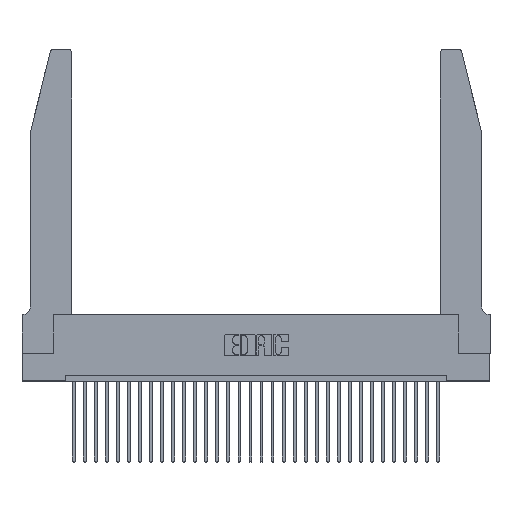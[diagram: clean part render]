
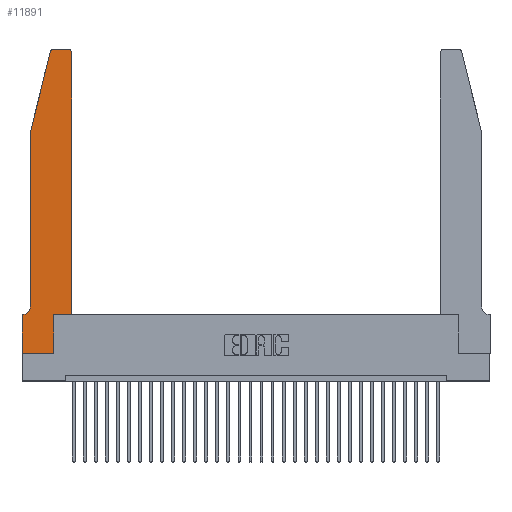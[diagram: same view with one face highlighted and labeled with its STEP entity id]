
A CAD part, top view. The second image highlights one B-rep face of the part: STEP entity #11891.
In plain terms, the highlighted planar face has unit normal (0, 0, 1).
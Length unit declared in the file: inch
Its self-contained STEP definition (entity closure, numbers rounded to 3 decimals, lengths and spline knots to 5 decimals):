
#624 = DIRECTION ( 'NONE',  ( 0., -1., 0. ) ) ;
#939 = EDGE_CURVE ( 'NONE', #3533, #28331, #27100, .T. ) ;
#1488 = EDGE_CURVE ( 'NONE', #28331, #21614, #12310, .T. ) ;
#1603 = VERTEX_POINT ( 'NONE', #28824 ) ;
#1718 = AXIS2_PLACEMENT_3D ( 'NONE', #11492, #25703, #21127 ) ;
#2092 = CARTESIAN_POINT ( 'NONE',  ( 0.0055, 0.35, 0.37 ) ) ;
#2944 = CARTESIAN_POINT ( 'NONE',  ( 0.4505, 0.35, 0.37 ) ) ;
#3262 = VECTOR ( 'NONE', #7074, 39.37008 ) ;
#3434 = AXIS2_PLACEMENT_3D ( 'NONE', #5565, #19455, #17740 ) ;
#3473 = CARTESIAN_POINT ( 'NONE',  ( 0.4505, 2.72, 0.37 ) ) ;
#3480 = ORIENTED_EDGE ( 'NONE', *, *, #20448, .T. ) ;
#3533 = VERTEX_POINT ( 'NONE', #3473 ) ;
#3697 = CARTESIAN_POINT ( 'NONE',  ( 0., 0.35, 0.37 ) ) ;
#4488 = VECTOR ( 'NONE', #15259, 39.37008 ) ;
#5148 = EDGE_CURVE ( 'NONE', #29528, #20978, #16228, .T. ) ;
#5565 = CARTESIAN_POINT ( 'NONE',  ( 0.0055, 0.42, 0.37 ) ) ;
#5737 = CARTESIAN_POINT ( 'NONE',  ( 0., 0., 0.37 ) ) ;
#6694 = ORIENTED_EDGE ( 'NONE', *, *, #939, .T. ) ;
#6777 = CIRCLE ( 'NONE', #3434, 0.07 ) ;
#6950 = EDGE_CURVE ( 'NONE', #27417, #1603, #30986, .T. ) ;
#7074 = DIRECTION ( 'NONE',  ( 0., 1., 0. ) ) ;
#7386 = CARTESIAN_POINT ( 'NONE',  ( 0.4505, 0.35, 0.37 ) ) ;
#7404 = ORIENTED_EDGE ( 'NONE', *, *, #1488, .T. ) ;
#7654 = CIRCLE ( 'NONE', #24157, 0.03 ) ;
#7812 = LINE ( 'NONE', #21998, #14275 ) ;
#8032 = ORIENTED_EDGE ( 'NONE', *, *, #24967, .T. ) ;
#8493 = ORIENTED_EDGE ( 'NONE', *, *, #16739, .T. ) ;
#8572 = CARTESIAN_POINT ( 'NONE',  ( 0.4205, 2.75, 0.37 ) ) ;
#8631 = LINE ( 'NONE', #7386, #3262 ) ;
#8802 = CARTESIAN_POINT ( 'NONE',  ( 0.284, 2.75, 0.37 ) ) ;
#8907 = VECTOR ( 'NONE', #25138, 39.37008 ) ;
#9282 = VERTEX_POINT ( 'NONE', #10250 ) ;
#9800 = EDGE_LOOP ( 'NONE', ( #7404, #21762, #13279, #27563, #30199, #23719, #8493, #3480, #22767, #8032, #12245, #6694 ) ) ;
#9854 = VECTOR ( 'NONE', #624, 39.37008 ) ;
#9991 = CARTESIAN_POINT ( 'NONE',  ( 0.0755, 2., 0.37 ) ) ;
#10250 = CARTESIAN_POINT ( 'NONE',  ( 0.25487, 2.72718, 0.37 ) ) ;
#11074 = CARTESIAN_POINT ( 'NONE',  ( 0.0755, 0.35, 0.37 ) ) ;
#11308 = CARTESIAN_POINT ( 'NONE',  ( 0., 0., 0.37 ) ) ;
#11477 = AXIS2_PLACEMENT_3D ( 'NONE', #28667, #11798, #26436 ) ;
#11492 = CARTESIAN_POINT ( 'NONE',  ( 0.4205, 2.72, 0.37 ) ) ;
#11588 = CARTESIAN_POINT ( 'NONE',  ( 0.284, 2.72, 0.37 ) ) ;
#11798 = DIRECTION ( 'NONE',  ( 0., 0., 1. ) ) ;
#11891 = ADVANCED_FACE ( 'NONE', ( #31187 ), #31394, .T. ) ;
#12128 = VECTOR ( 'NONE', #30871, 39.37008 ) ;
#12245 = ORIENTED_EDGE ( 'NONE', *, *, #24285, .T. ) ;
#12310 = LINE ( 'NONE', #27388, #8907 ) ;
#12819 = VECTOR ( 'NONE', #28152, 39.37008 ) ;
#13279 = ORIENTED_EDGE ( 'NONE', *, *, #23619, .T. ) ;
#13981 = LINE ( 'NONE', #11074, #12819 ) ;
#14224 = CARTESIAN_POINT ( 'NONE',  ( 0.0755, 2., 0.37 ) ) ;
#14275 = VECTOR ( 'NONE', #14578, 39.37008 ) ;
#14578 = DIRECTION ( 'NONE',  ( 1., 0., 0. ) ) ;
#14984 = VERTEX_POINT ( 'NONE', #2092 ) ;
#15259 = DIRECTION ( 'NONE',  ( -0.239, -0.971, 0. ) ) ;
#15843 = LINE ( 'NONE', #9991, #4488 ) ;
#16228 = LINE ( 'NONE', #14224, #12128 ) ;
#16281 = LINE ( 'NONE', #5737, #9854 ) ;
#16739 = EDGE_CURVE ( 'NONE', #27795, #19474, #16281, .T. ) ;
#17278 = EDGE_CURVE ( 'NONE', #21614, #9282, #7654, .T. ) ;
#17740 = DIRECTION ( 'NONE',  ( -1., 0., 0. ) ) ;
#18442 = DIRECTION ( 'NONE',  ( 0., 1., 0. ) ) ;
#19332 = VECTOR ( 'NONE', #19713, 39.37008 ) ;
#19455 = DIRECTION ( 'NONE',  ( 0., 0., -1. ) ) ;
#19474 = VERTEX_POINT ( 'NONE', #11308 ) ;
#19713 = DIRECTION ( 'NONE',  ( 1., 0., 0. ) ) ;
#19762 = EDGE_CURVE ( 'NONE', #20978, #14984, #6777, .T. ) ;
#20448 = EDGE_CURVE ( 'NONE', #19474, #27417, #30721, .T. ) ;
#20576 = CARTESIAN_POINT ( 'NONE',  ( 0.0755, 2., 0.37 ) ) ;
#20978 = VERTEX_POINT ( 'NONE', #25087 ) ;
#21127 = DIRECTION ( 'NONE',  ( 1., 0., 0. ) ) ;
#21462 = CARTESIAN_POINT ( 'NONE',  ( 0.2865, 0., 0.37 ) ) ;
#21614 = VERTEX_POINT ( 'NONE', #8802 ) ;
#21762 = ORIENTED_EDGE ( 'NONE', *, *, #17278, .T. ) ;
#21998 = CARTESIAN_POINT ( 'NONE',  ( 0.4505, 0.35, 0.37 ) ) ;
#22229 = VECTOR ( 'NONE', #18442, 39.37008 ) ;
#22767 = ORIENTED_EDGE ( 'NONE', *, *, #6950, .T. ) ;
#23619 = EDGE_CURVE ( 'NONE', #9282, #29528, #15843, .T. ) ;
#23719 = ORIENTED_EDGE ( 'NONE', *, *, #27252, .T. ) ;
#23792 = DIRECTION ( 'NONE',  ( 1., 0., 0. ) ) ;
#24157 = AXIS2_PLACEMENT_3D ( 'NONE', #11588, #30991, #23792 ) ;
#24285 = EDGE_CURVE ( 'NONE', #28200, #3533, #8631, .T. ) ;
#24967 = EDGE_CURVE ( 'NONE', #1603, #28200, #7812, .T. ) ;
#25087 = CARTESIAN_POINT ( 'NONE',  ( 0.0755, 0.42, 0.37 ) ) ;
#25138 = DIRECTION ( 'NONE',  ( -1., 0., 0. ) ) ;
#25703 = DIRECTION ( 'NONE',  ( 0., 0., 1. ) ) ;
#26436 = DIRECTION ( 'NONE',  ( 1., 0., 0. ) ) ;
#27100 = CIRCLE ( 'NONE', #1718, 0.03 ) ;
#27240 = CARTESIAN_POINT ( 'NONE',  ( 0., 0., 0.37 ) ) ;
#27252 = EDGE_CURVE ( 'NONE', #14984, #27795, #13981, .T. ) ;
#27388 = CARTESIAN_POINT ( 'NONE',  ( 0.2605, 2.75, 0.37 ) ) ;
#27417 = VERTEX_POINT ( 'NONE', #21462 ) ;
#27563 = ORIENTED_EDGE ( 'NONE', *, *, #5148, .T. ) ;
#27795 = VERTEX_POINT ( 'NONE', #3697 ) ;
#28152 = DIRECTION ( 'NONE',  ( -1., 0., 0. ) ) ;
#28200 = VERTEX_POINT ( 'NONE', #2944 ) ;
#28331 = VERTEX_POINT ( 'NONE', #8572 ) ;
#28667 = CARTESIAN_POINT ( 'NONE',  ( 0., 0.35, 0.37 ) ) ;
#28824 = CARTESIAN_POINT ( 'NONE',  ( 0.2865, 0.35, 0.37 ) ) ;
#29528 = VERTEX_POINT ( 'NONE', #20576 ) ;
#30199 = ORIENTED_EDGE ( 'NONE', *, *, #19762, .T. ) ;
#30670 = CARTESIAN_POINT ( 'NONE',  ( 0.2865, 0.35, 0.37 ) ) ;
#30721 = LINE ( 'NONE', #27240, #19332 ) ;
#30871 = DIRECTION ( 'NONE',  ( 0., -1., 0. ) ) ;
#30986 = LINE ( 'NONE', #30670, #22229 ) ;
#30991 = DIRECTION ( 'NONE',  ( 0., 0., 1. ) ) ;
#31187 = FACE_OUTER_BOUND ( 'NONE', #9800, .T. ) ;
#31394 = PLANE ( 'NONE',  #11477 ) ;
